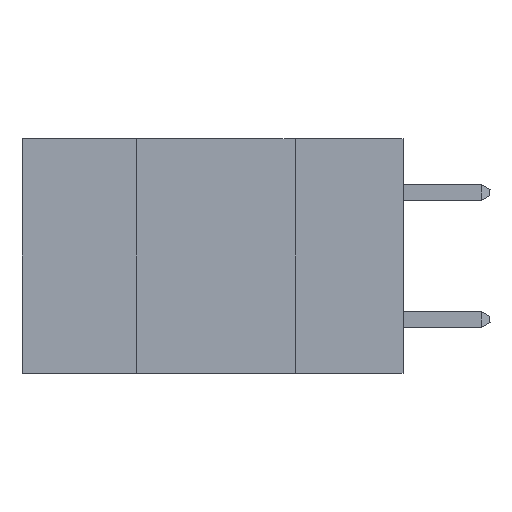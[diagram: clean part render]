
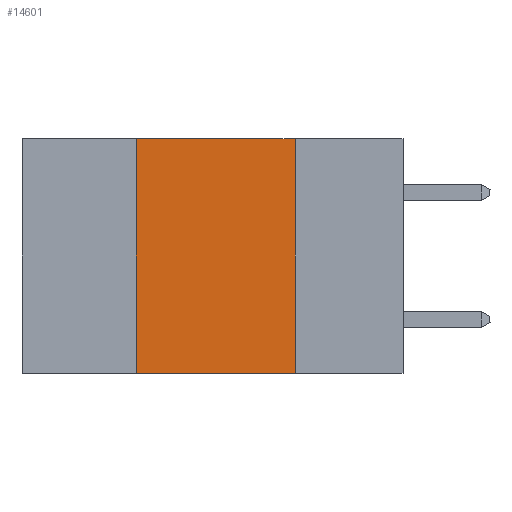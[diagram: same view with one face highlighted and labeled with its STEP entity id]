
A CAD part, left-side view. The second image highlights one B-rep face of the part: STEP entity #14601.
In plain terms, the highlighted planar face has unit normal (-1, 0, 0).
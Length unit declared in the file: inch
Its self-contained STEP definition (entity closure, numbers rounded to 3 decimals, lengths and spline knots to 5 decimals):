
#1003 = DIRECTION ( 'NONE',  ( 0., 0., -1. ) ) ;
#1235 = CARTESIAN_POINT ( 'NONE',  ( 0., 0.6, -0.37 ) ) ;
#1898 = LINE ( 'NONE', #1235, #22134 ) ;
#2872 = CARTESIAN_POINT ( 'NONE',  ( 0., 0.17, -0.37 ) ) ;
#3229 = CARTESIAN_POINT ( 'NONE',  ( 0., 0.42, 0. ) ) ;
#3302 = VERTEX_POINT ( 'NONE', #2872 ) ;
#3613 = LINE ( 'NONE', #20083, #8912 ) ;
#3948 = DIRECTION ( 'NONE',  ( 0., 0., -1. ) ) ;
#6543 = VECTOR ( 'NONE', #9248, 39.37008 ) ;
#6854 = EDGE_CURVE ( 'NONE', #13365, #21835, #3613, .T. ) ;
#8570 = CARTESIAN_POINT ( 'NONE',  ( 0., 0.42, -0.37 ) ) ;
#8912 = VECTOR ( 'NONE', #10439, 39.37008 ) ;
#9011 = EDGE_LOOP ( 'NONE', ( #17720, #11339, #10954, #24096 ) ) ;
#9207 = EDGE_CURVE ( 'NONE', #24373, #3302, #1898, .T. ) ;
#9248 = DIRECTION ( 'NONE',  ( 0., 0., 1. ) ) ;
#10439 = DIRECTION ( 'NONE',  ( 0., -1., 0. ) ) ;
#10634 = EDGE_CURVE ( 'NONE', #24373, #13365, #17599, .T. ) ;
#10954 = ORIENTED_EDGE ( 'NONE', *, *, #10634, .F. ) ;
#11339 = ORIENTED_EDGE ( 'NONE', *, *, #6854, .F. ) ;
#12984 = DIRECTION ( 'NONE',  ( 1., 0., 0. ) ) ;
#13365 = VERTEX_POINT ( 'NONE', #20583 ) ;
#13974 = LINE ( 'NONE', #17641, #23515 ) ;
#14190 = CARTESIAN_POINT ( 'NONE',  ( 0., 0.17, 0. ) ) ;
#14601 = ADVANCED_FACE ( 'NONE', ( #21755 ), #14844, .F. ) ;
#14844 = PLANE ( 'NONE',  #24819 ) ;
#17599 = LINE ( 'NONE', #3229, #6543 ) ;
#17641 = CARTESIAN_POINT ( 'NONE',  ( 0., 0.17, 0. ) ) ;
#17720 = ORIENTED_EDGE ( 'NONE', *, *, #24172, .F. ) ;
#20083 = CARTESIAN_POINT ( 'NONE',  ( 0., 0.6, 0. ) ) ;
#20583 = CARTESIAN_POINT ( 'NONE',  ( 0., 0.42, 0. ) ) ;
#20912 = DIRECTION ( 'NONE',  ( 0., -1., 0. ) ) ;
#21755 = FACE_OUTER_BOUND ( 'NONE', #9011, .T. ) ;
#21835 = VERTEX_POINT ( 'NONE', #14190 ) ;
#22134 = VECTOR ( 'NONE', #20912, 39.37008 ) ;
#22520 = CARTESIAN_POINT ( 'NONE',  ( 0., 0.6, 0. ) ) ;
#23515 = VECTOR ( 'NONE', #3948, 39.37008 ) ;
#24096 = ORIENTED_EDGE ( 'NONE', *, *, #9207, .T. ) ;
#24172 = EDGE_CURVE ( 'NONE', #21835, #3302, #13974, .T. ) ;
#24373 = VERTEX_POINT ( 'NONE', #8570 ) ;
#24819 = AXIS2_PLACEMENT_3D ( 'NONE', #22520, #12984, #1003 ) ;
